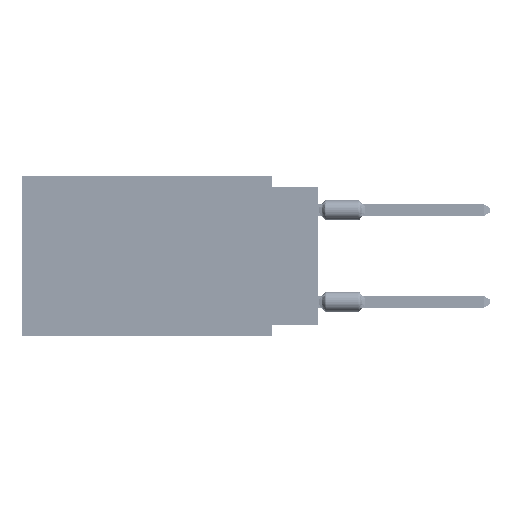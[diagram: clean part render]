
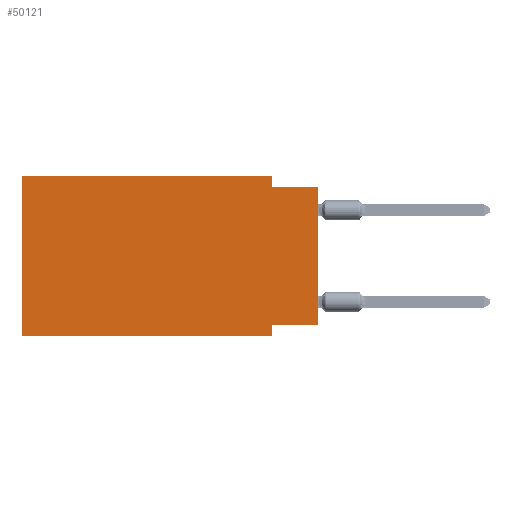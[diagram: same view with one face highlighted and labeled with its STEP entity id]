
A CAD part, left-side view. The second image highlights one B-rep face of the part: STEP entity #50121.
In plain terms, the highlighted planar face has unit normal (-1, 0, 0).
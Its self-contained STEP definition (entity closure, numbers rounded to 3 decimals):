
#975 = CARTESIAN_POINT ( 'NONE',  ( 0., 16.383, 0. ) ) ;
#2974 = CARTESIAN_POINT ( 'NONE',  ( 0., 0., -8.255 ) ) ;
#5783 = CARTESIAN_POINT ( 'NONE',  ( 0., 16.383, 0. ) ) ;
#6043 = EDGE_CURVE ( 'NONE', #47650, #36541, #35759, .T. ) ;
#6709 = ORIENTED_EDGE ( 'NONE', *, *, #47373, .F. ) ;
#8081 = LINE ( 'NONE', #48778, #19368 ) ;
#9072 = VERTEX_POINT ( 'NONE', #28122 ) ;
#9580 = CARTESIAN_POINT ( 'NONE',  ( 0., 16.383, 0. ) ) ;
#10522 = VECTOR ( 'NONE', #10977, 1000. ) ;
#10977 = DIRECTION ( 'NONE',  ( 0., -1., 0. ) ) ;
#11402 = ORIENTED_EDGE ( 'NONE', *, *, #43324, .F. ) ;
#13324 = DIRECTION ( 'NONE',  ( 0., 0., 1. ) ) ;
#14349 = CARTESIAN_POINT ( 'NONE',  ( 0., 2.54, -8.89 ) ) ;
#15014 = LINE ( 'NONE', #14349, #41046 ) ;
#15096 = ORIENTED_EDGE ( 'NONE', *, *, #50483, .F. ) ;
#19368 = VECTOR ( 'NONE', #64172, 1000. ) ;
#19437 = LINE ( 'NONE', #5783, #42631 ) ;
#19811 = DIRECTION ( 'NONE',  ( 0., 0., -1. ) ) ;
#22536 = EDGE_CURVE ( 'NONE', #53820, #27514, #58144, .T. ) ;
#24310 = EDGE_CURVE ( 'NONE', #28772, #58232, #8081, .T. ) ;
#24411 = VECTOR ( 'NONE', #31993, 1000. ) ;
#25204 = DIRECTION ( 'NONE',  ( 0., 1., 0. ) ) ;
#27514 = VERTEX_POINT ( 'NONE', #56534 ) ;
#28122 = CARTESIAN_POINT ( 'NONE',  ( 0., 2.54, -8.255 ) ) ;
#28278 = VECTOR ( 'NONE', #53004, 1000. ) ;
#28772 = VERTEX_POINT ( 'NONE', #31050 ) ;
#31050 = CARTESIAN_POINT ( 'NONE',  ( 0., 16.383, -8.89 ) ) ;
#31993 = DIRECTION ( 'NONE',  ( 0., 0., 1. ) ) ;
#32993 = AXIS2_PLACEMENT_3D ( 'NONE', #66316, #51645, #19811 ) ;
#35759 = LINE ( 'NONE', #58001, #24411 ) ;
#36541 = VERTEX_POINT ( 'NONE', #61420 ) ;
#36962 = LINE ( 'NONE', #57848, #10522 ) ;
#38908 = EDGE_LOOP ( 'NONE', ( #48985, #41250, #45918, #44958, #11402, #64251, #6709, #15096 ) ) ;
#40340 = DIRECTION ( 'NONE',  ( 0., 0., -1. ) ) ;
#40431 = EDGE_CURVE ( 'NONE', #41047, #53820, #19437, .T. ) ;
#40662 = VECTOR ( 'NONE', #25204, 1000. ) ;
#41046 = VECTOR ( 'NONE', #40340, 1000. ) ;
#41047 = VERTEX_POINT ( 'NONE', #975 ) ;
#41250 = ORIENTED_EDGE ( 'NONE', *, *, #48612, .F. ) ;
#41945 = CARTESIAN_POINT ( 'NONE',  ( 0., 2.54, -8.89 ) ) ;
#42631 = VECTOR ( 'NONE', #47485, 1000. ) ;
#43324 = EDGE_CURVE ( 'NONE', #28772, #41047, #56447, .T. ) ;
#44958 = ORIENTED_EDGE ( 'NONE', *, *, #40431, .F. ) ;
#45918 = ORIENTED_EDGE ( 'NONE', *, *, #22536, .F. ) ;
#46158 = FACE_OUTER_BOUND ( 'NONE', #38908, .T. ) ;
#47373 = EDGE_CURVE ( 'NONE', #9072, #58232, #15014, .T. ) ;
#47485 = DIRECTION ( 'NONE',  ( 0., -1., 0. ) ) ;
#47650 = VERTEX_POINT ( 'NONE', #64228 ) ;
#48425 = VECTOR ( 'NONE', #13324, 1000. ) ;
#48612 = EDGE_CURVE ( 'NONE', #27514, #36541, #36962, .T. ) ;
#48778 = CARTESIAN_POINT ( 'NONE',  ( 0., 16.383, -8.89 ) ) ;
#48985 = ORIENTED_EDGE ( 'NONE', *, *, #6043, .T. ) ;
#50121 = ADVANCED_FACE ( 'NONE', ( #46158 ), #50614, .F. ) ;
#50483 = EDGE_CURVE ( 'NONE', #47650, #9072, #66240, .T. ) ;
#50614 = PLANE ( 'NONE',  #32993 ) ;
#51645 = DIRECTION ( 'NONE',  ( 1., 0., 0. ) ) ;
#53004 = DIRECTION ( 'NONE',  ( 0., 0., -1. ) ) ;
#53820 = VERTEX_POINT ( 'NONE', #60676 ) ;
#56447 = LINE ( 'NONE', #9580, #48425 ) ;
#56534 = CARTESIAN_POINT ( 'NONE',  ( 0., 2.54, -0.635 ) ) ;
#57137 = CARTESIAN_POINT ( 'NONE',  ( 0., 2.54, 0. ) ) ;
#57848 = CARTESIAN_POINT ( 'NONE',  ( 0., 0., -0.635 ) ) ;
#58001 = CARTESIAN_POINT ( 'NONE',  ( 0., 0., 0. ) ) ;
#58144 = LINE ( 'NONE', #57137, #28278 ) ;
#58232 = VERTEX_POINT ( 'NONE', #41945 ) ;
#60676 = CARTESIAN_POINT ( 'NONE',  ( 0., 2.54, 0. ) ) ;
#61420 = CARTESIAN_POINT ( 'NONE',  ( 0., 0., -0.635 ) ) ;
#64172 = DIRECTION ( 'NONE',  ( 0., -1., 0. ) ) ;
#64228 = CARTESIAN_POINT ( 'NONE',  ( 0., 0., -8.255 ) ) ;
#64251 = ORIENTED_EDGE ( 'NONE', *, *, #24310, .T. ) ;
#66240 = LINE ( 'NONE', #2974, #40662 ) ;
#66316 = CARTESIAN_POINT ( 'NONE',  ( 0., 16.383, 0. ) ) ;
